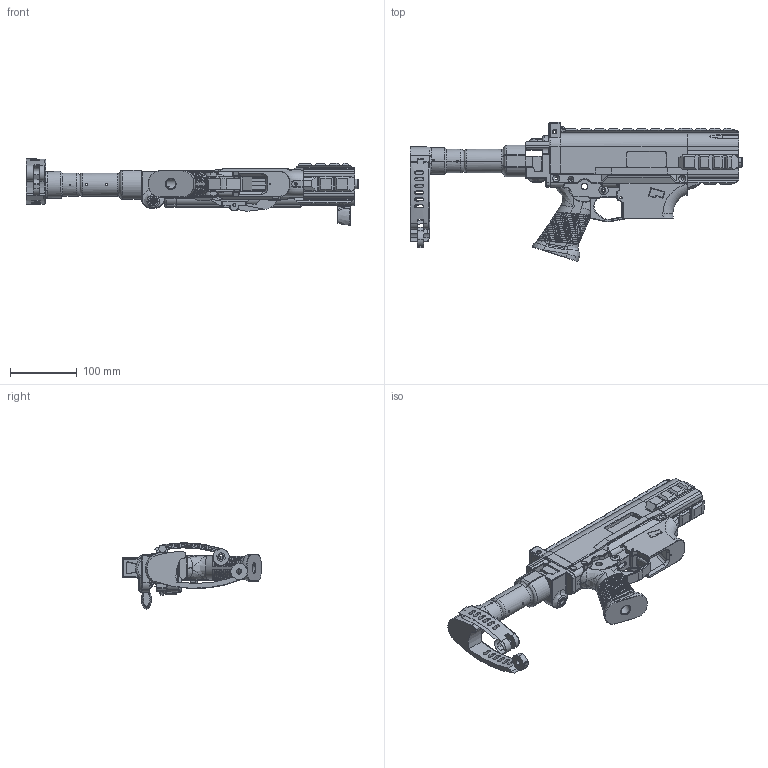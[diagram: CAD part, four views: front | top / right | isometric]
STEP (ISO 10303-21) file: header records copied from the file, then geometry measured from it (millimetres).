
FILE_DESCRIPTION (( 'STEP AP203' ), '1' );
FILE_NAME ('Assembly for refference only.STEP', '2020-09-09T05:31:06', ( '' ), ( '' ), 'SwSTEP 2.0', 'SolidWorks 2019', '' );
FILE_SCHEMA (( 'CONFIG_CONTROL_DESIGN' ));
Length unit declared in the file: millimetre
Products named in the file (22): carbon arrow; lower bolt; upper bolt.stp; MOD9_magwell.step; MOD9_barrel_retainer.step; tailhook brace final.stp; MOD9_charging_handle.step; MOD9_upper_receiver.step; Assembly for refference only; MOD9_ejector.step; MOD9_pistol_grip.step; MOD9_mag_catch.step; MOD9_bolt_housing.step; MOD9_endcap.step; MOD9_threaded_stock_adapter; bolt assy; Lauf_Standard; MOD9_feed_ramp.step; MOD9_lower_receiver.step; firing pin; MOD9_G36_stock_lock.step; MOD9_ejector_mount.step
Assembly tree (21 placements, depth 3):
  Assembly for refference only
    MOD9_barrel_retainer.step
    MOD9_bolt_housing.step
    MOD9_charging_handle.step
    MOD9_ejector.step
    MOD9_ejector_mount.step
    MOD9_endcap.step
    MOD9_feed_ramp.step
    MOD9_G36_stock_lock.step
    MOD9_lower_receiver.step
    MOD9_mag_catch.step
    MOD9_magwell.step
    MOD9_pistol_grip.step
    MOD9_upper_receiver.step
    carbon arrow
    bolt assy
      lower bolt
      upper bolt.stp
    firing pin
    Lauf_Standard
    MOD9_threaded_stock_adapter
    tailhook brace final.stp
Bounding box: 497.99 x 208.54 x 99.29 mm (x, y, z)
Volume: 1008792.3 mm3; surface area: 384389.7 mm2
Topology: 20 solids, 23 shells, 4102 faces, 11058 edges, 6993 vertices
Faces by surface type: plane 1766, cylinder 1157, bspline 792, cone 232, torus 111, sphere 44
Entity records: 189643 total; most frequent: CARTESIAN_POINT 93439, ORIENTED_EDGE 22016, DIRECTION 15765, EDGE_CURVE 11014, VERTEX_POINT 6993, VECTOR 5457, LINE 5457, AXIS2_PLACEMENT_3D 5154
